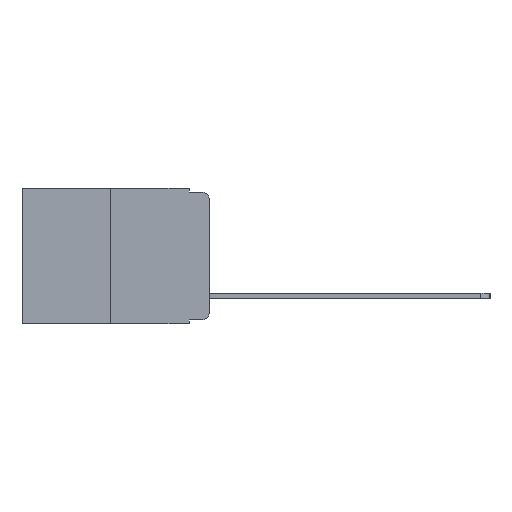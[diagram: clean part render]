
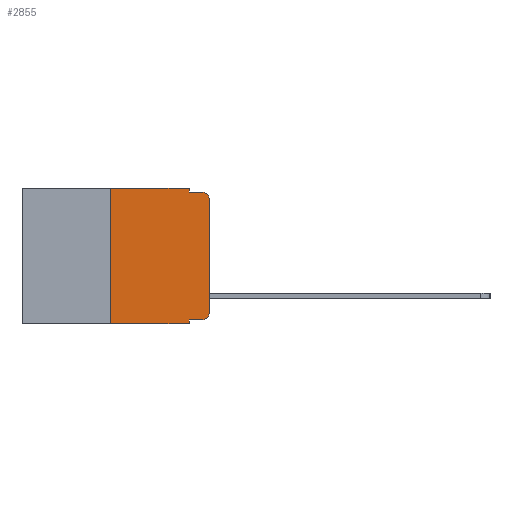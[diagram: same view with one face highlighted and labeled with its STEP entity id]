
A CAD part, left-side view. The second image highlights one B-rep face of the part: STEP entity #2855.
In plain terms, the highlighted planar face has unit normal (-1, 0, 0).
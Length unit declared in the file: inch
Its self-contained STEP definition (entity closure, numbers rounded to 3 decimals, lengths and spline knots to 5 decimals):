
#107 = CARTESIAN_POINT ( 'NONE',  ( 0., 0.473, 0. ) ) ;
#177 = CARTESIAN_POINT ( 'NONE',  ( 0., 0.473, -0.343 ) ) ;
#531 = VECTOR ( 'NONE', #16252, 39.37008 ) ;
#665 = VERTEX_POINT ( 'NONE', #4417 ) ;
#823 = CARTESIAN_POINT ( 'NONE',  ( 0., 0.02, -0.313 ) ) ;
#936 = VERTEX_POINT ( 'NONE', #11134 ) ;
#1331 = CARTESIAN_POINT ( 'NONE',  ( 0., 0.25, 0. ) ) ;
#1938 = CARTESIAN_POINT ( 'NONE',  ( 0., 0.051, 0. ) ) ;
#1975 = DIRECTION ( 'NONE',  ( 0., 0., -1. ) ) ;
#2058 = LINE ( 'NONE', #177, #15153 ) ;
#2188 = VERTEX_POINT ( 'NONE', #6444 ) ;
#2202 = DIRECTION ( 'NONE',  ( 0., 0., -1. ) ) ;
#2281 = VECTOR ( 'NONE', #10681, 39.37008 ) ;
#2363 = ORIENTED_EDGE ( 'NONE', *, *, #4690, .T. ) ;
#2747 = AXIS2_PLACEMENT_3D ( 'NONE', #823, #10312, #2202 ) ;
#2855 = ADVANCED_FACE ( 'NONE', ( #9343 ), #10877, .F. ) ;
#3051 = DIRECTION ( 'NONE',  ( 0., -1., 0. ) ) ;
#3812 = DIRECTION ( 'NONE',  ( -1., 0., 0. ) ) ;
#3944 = AXIS2_PLACEMENT_3D ( 'NONE', #6186, #10954, #1975 ) ;
#4257 = LINE ( 'NONE', #11766, #531 ) ;
#4417 = CARTESIAN_POINT ( 'NONE',  ( 0., 0.25, -0.343 ) ) ;
#4690 = EDGE_CURVE ( 'NONE', #10631, #15857, #14218, .T. ) ;
#4811 = VERTEX_POINT ( 'NONE', #14101 ) ;
#5646 = CARTESIAN_POINT ( 'NONE',  ( 0., 0.051, -0.333 ) ) ;
#6186 = CARTESIAN_POINT ( 'NONE',  ( 0., 0.473, 0. ) ) ;
#6352 = CARTESIAN_POINT ( 'NONE',  ( 0., 0.25, 0. ) ) ;
#6444 = CARTESIAN_POINT ( 'NONE',  ( 0., 0.051, -0.01 ) ) ;
#7176 = LINE ( 'NONE', #8859, #16202 ) ;
#7257 = ORIENTED_EDGE ( 'NONE', *, *, #13405, .T. ) ;
#7334 = AXIS2_PLACEMENT_3D ( 'NONE', #11692, #3812, #12844 ) ;
#7540 = EDGE_CURVE ( 'NONE', #4811, #10631, #12440, .T. ) ;
#7671 = ORIENTED_EDGE ( 'NONE', *, *, #8440, .F. ) ;
#7821 = ORIENTED_EDGE ( 'NONE', *, *, #15431, .T. ) ;
#7824 = VECTOR ( 'NONE', #12151, 39.37008 ) ;
#8102 = ORIENTED_EDGE ( 'NONE', *, *, #7540, .T. ) ;
#8440 = EDGE_CURVE ( 'NONE', #4811, #16057, #15687, .T. ) ;
#8548 = EDGE_CURVE ( 'NONE', #15084, #10445, #11118, .T. ) ;
#8667 = LINE ( 'NONE', #1938, #14864 ) ;
#8859 = CARTESIAN_POINT ( 'NONE',  ( 0., 0.051, -0.01 ) ) ;
#9209 = CARTESIAN_POINT ( 'NONE',  ( 0., 0.02, -0.333 ) ) ;
#9244 = VECTOR ( 'NONE', #3051, 39.37008 ) ;
#9343 = FACE_OUTER_BOUND ( 'NONE', #16292, .T. ) ;
#10054 = EDGE_CURVE ( 'NONE', #665, #15084, #14031, .T. ) ;
#10312 = DIRECTION ( 'NONE',  ( -1., 0., 0. ) ) ;
#10445 = VERTEX_POINT ( 'NONE', #13648 ) ;
#10631 = VERTEX_POINT ( 'NONE', #9209 ) ;
#10681 = DIRECTION ( 'NONE',  ( 0., 0., -1. ) ) ;
#10877 = PLANE ( 'NONE',  #3944 ) ;
#10954 = DIRECTION ( 'NONE',  ( 1., 0., 0. ) ) ;
#10988 = VECTOR ( 'NONE', #13117, 39.37008 ) ;
#11010 = DIRECTION ( 'NONE',  ( 0., -1., 0. ) ) ;
#11095 = CARTESIAN_POINT ( 'NONE',  ( 0., 0.02, -0.01 ) ) ;
#11118 = LINE ( 'NONE', #107, #7824 ) ;
#11134 = CARTESIAN_POINT ( 'NONE',  ( 0., 0., -0.03 ) ) ;
#11546 = ORIENTED_EDGE ( 'NONE', *, *, #8548, .F. ) ;
#11550 = VERTEX_POINT ( 'NONE', #11095 ) ;
#11687 = EDGE_CURVE ( 'NONE', #10445, #2188, #8667, .T. ) ;
#11692 = CARTESIAN_POINT ( 'NONE',  ( 0., 0.02, -0.03 ) ) ;
#11766 = CARTESIAN_POINT ( 'NONE',  ( 0., 0., 0. ) ) ;
#12151 = DIRECTION ( 'NONE',  ( 0., -1., 0. ) ) ;
#12440 = LINE ( 'NONE', #5646, #9244 ) ;
#12465 = EDGE_CURVE ( 'NONE', #2188, #11550, #7176, .T. ) ;
#12487 = DIRECTION ( 'NONE',  ( 0., 0., -1. ) ) ;
#12844 = DIRECTION ( 'NONE',  ( 0., 0., -1. ) ) ;
#13117 = DIRECTION ( 'NONE',  ( 0., 0., 1. ) ) ;
#13224 = CARTESIAN_POINT ( 'NONE',  ( 0., 0., -0.313 ) ) ;
#13405 = EDGE_CURVE ( 'NONE', #665, #16057, #2058, .T. ) ;
#13648 = CARTESIAN_POINT ( 'NONE',  ( 0., 0.051, 0. ) ) ;
#13854 = ORIENTED_EDGE ( 'NONE', *, *, #11687, .F. ) ;
#13958 = EDGE_CURVE ( 'NONE', #936, #11550, #15871, .T. ) ;
#14031 = LINE ( 'NONE', #1331, #10988 ) ;
#14101 = CARTESIAN_POINT ( 'NONE',  ( 0., 0.051, -0.333 ) ) ;
#14162 = CARTESIAN_POINT ( 'NONE',  ( 0., 0.051, 0. ) ) ;
#14170 = ORIENTED_EDGE ( 'NONE', *, *, #12465, .F. ) ;
#14218 = CIRCLE ( 'NONE', #2747, 0.02 ) ;
#14523 = CARTESIAN_POINT ( 'NONE',  ( 0., 0.051, -0.343 ) ) ;
#14864 = VECTOR ( 'NONE', #12487, 39.37008 ) ;
#15084 = VERTEX_POINT ( 'NONE', #6352 ) ;
#15153 = VECTOR ( 'NONE', #11010, 39.37008 ) ;
#15189 = ORIENTED_EDGE ( 'NONE', *, *, #13958, .T. ) ;
#15431 = EDGE_CURVE ( 'NONE', #15857, #936, #4257, .T. ) ;
#15687 = LINE ( 'NONE', #14162, #2281 ) ;
#15767 = DIRECTION ( 'NONE',  ( 0., -1., 0. ) ) ;
#15857 = VERTEX_POINT ( 'NONE', #13224 ) ;
#15871 = CIRCLE ( 'NONE', #7334, 0.02 ) ;
#16057 = VERTEX_POINT ( 'NONE', #14523 ) ;
#16202 = VECTOR ( 'NONE', #15767, 39.37008 ) ;
#16252 = DIRECTION ( 'NONE',  ( 0., 0., 1. ) ) ;
#16263 = ORIENTED_EDGE ( 'NONE', *, *, #10054, .F. ) ;
#16292 = EDGE_LOOP ( 'NONE', ( #7821, #15189, #14170, #13854, #11546, #16263, #7257, #7671, #8102, #2363 ) ) ;
